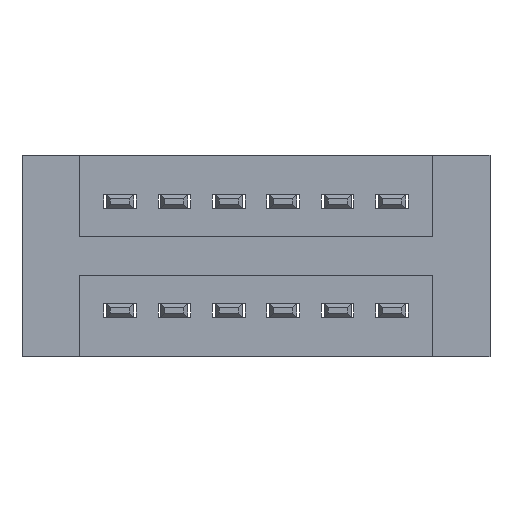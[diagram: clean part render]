
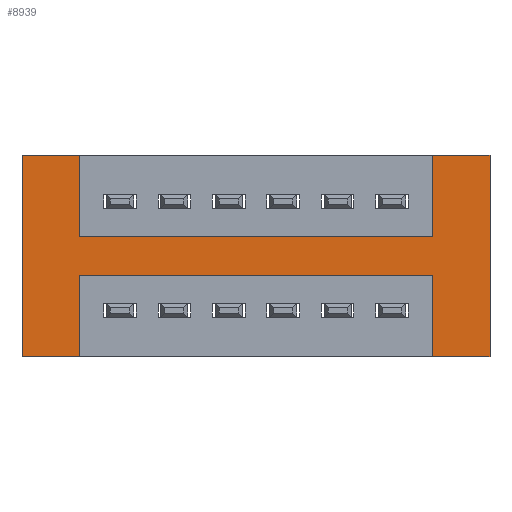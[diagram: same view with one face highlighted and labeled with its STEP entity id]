
A CAD part, front view. The second image highlights one B-rep face of the part: STEP entity #8939.
In plain terms, the highlighted planar face has unit normal (0, -1, 0).
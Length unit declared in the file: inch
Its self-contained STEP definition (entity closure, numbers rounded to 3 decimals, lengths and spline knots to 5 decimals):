
#86 = DIRECTION ( 'NONE',  ( 0., 0., -1. ) ) ;
#334 = DIRECTION ( 'NONE',  ( -1., 0., 0. ) ) ;
#479 = CARTESIAN_POINT ( 'NONE',  ( 0.3925, 0., -0.22 ) ) ;
#517 = VECTOR ( 'NONE', #3859, 39.37008 ) ;
#543 = ORIENTED_EDGE ( 'NONE', *, *, #7268, .F. ) ;
#548 = VECTOR ( 'NONE', #3588, 39.37008 ) ;
#1015 = VERTEX_POINT ( 'NONE', #8087 ) ;
#1110 = VERTEX_POINT ( 'NONE', #8718 ) ;
#1115 = VERTEX_POINT ( 'NONE', #8397 ) ;
#1174 = EDGE_CURVE ( 'NONE', #3664, #2440, #4881, .T. ) ;
#1403 = DIRECTION ( 'NONE',  ( 1., 0., 0. ) ) ;
#1459 = CARTESIAN_POINT ( 'NONE',  ( 1.0425, 0., -0.15 ) ) ;
#1495 = DIRECTION ( 'NONE',  ( 0., 0., 1. ) ) ;
#1603 = LINE ( 'NONE', #7203, #3324 ) ;
#1618 = LINE ( 'NONE', #4018, #8876 ) ;
#1695 = EDGE_CURVE ( 'NONE', #1115, #5210, #6433, .T. ) ;
#1724 = VERTEX_POINT ( 'NONE', #1761 ) ;
#1759 = DIRECTION ( 'NONE',  ( 0., 0., 1. ) ) ;
#1761 = CARTESIAN_POINT ( 'NONE',  ( 0.3925, 0., -0.37 ) ) ;
#1949 = EDGE_CURVE ( 'NONE', #2984, #5186, #8240, .T. ) ;
#2087 = EDGE_CURVE ( 'NONE', #5186, #4849, #5267, .T. ) ;
#2100 = VECTOR ( 'NONE', #8294, 39.37008 ) ;
#2111 = LINE ( 'NONE', #3970, #517 ) ;
#2144 = PLANE ( 'NONE',  #7568 ) ;
#2212 = VECTOR ( 'NONE', #3057, 39.37008 ) ;
#2410 = CARTESIAN_POINT ( 'NONE',  ( 0.3925, 0., -0.37 ) ) ;
#2432 = LINE ( 'NONE', #2410, #2212 ) ;
#2440 = VERTEX_POINT ( 'NONE', #5871 ) ;
#2491 = ORIENTED_EDGE ( 'NONE', *, *, #7507, .F. ) ;
#2665 = VERTEX_POINT ( 'NONE', #4403 ) ;
#2682 = CARTESIAN_POINT ( 'NONE',  ( 1.0425, 0., 0. ) ) ;
#2783 = CARTESIAN_POINT ( 'NONE',  ( 1.1475, 0., 0. ) ) ;
#2894 = DIRECTION ( 'NONE',  ( -1., 0., 0. ) ) ;
#2984 = VERTEX_POINT ( 'NONE', #5282 ) ;
#3057 = DIRECTION ( 'NONE',  ( 0., 0., -1. ) ) ;
#3156 = VECTOR ( 'NONE', #9092, 39.37008 ) ;
#3324 = VECTOR ( 'NONE', #2894, 39.37008 ) ;
#3435 = LINE ( 'NONE', #5165, #7123 ) ;
#3456 = ORIENTED_EDGE ( 'NONE', *, *, #1695, .T. ) ;
#3588 = DIRECTION ( 'NONE',  ( 0., 0., -1. ) ) ;
#3597 = CARTESIAN_POINT ( 'NONE',  ( 0., 0., -0.37 ) ) ;
#3601 = ORIENTED_EDGE ( 'NONE', *, *, #1174, .F. ) ;
#3664 = VERTEX_POINT ( 'NONE', #6521 ) ;
#3859 = DIRECTION ( 'NONE',  ( -1., 0., 0. ) ) ;
#3878 = CARTESIAN_POINT ( 'NONE',  ( 0.2875, 0., 0. ) ) ;
#3962 = VERTEX_POINT ( 'NONE', #2783 ) ;
#3970 = CARTESIAN_POINT ( 'NONE',  ( 0., 0., -0.37 ) ) ;
#4006 = LINE ( 'NONE', #7448, #2100 ) ;
#4018 = CARTESIAN_POINT ( 'NONE',  ( 0., 0., 0. ) ) ;
#4068 = EDGE_CURVE ( 'NONE', #2665, #3962, #3435, .T. ) ;
#4316 = EDGE_CURVE ( 'NONE', #1015, #1110, #1603, .T. ) ;
#4321 = DIRECTION ( 'NONE',  ( 0., 0., -1. ) ) ;
#4389 = VECTOR ( 'NONE', #86, 39.37008 ) ;
#4403 = CARTESIAN_POINT ( 'NONE',  ( 1.0425, 0., 0. ) ) ;
#4555 = CARTESIAN_POINT ( 'NONE',  ( 0.3925, 0., 0. ) ) ;
#4571 = ORIENTED_EDGE ( 'NONE', *, *, #8590, .T. ) ;
#4849 = VERTEX_POINT ( 'NONE', #1459 ) ;
#4881 = LINE ( 'NONE', #479, #6021 ) ;
#4915 = ORIENTED_EDGE ( 'NONE', *, *, #4316, .F. ) ;
#5067 = ORIENTED_EDGE ( 'NONE', *, *, #7570, .F. ) ;
#5124 = LINE ( 'NONE', #6022, #7116 ) ;
#5126 = EDGE_LOOP ( 'NONE', ( #4571, #5311, #7017, #7155, #8003, #5067, #3456, #6161, #543, #3601, #2491, #4915 ) ) ;
#5165 = CARTESIAN_POINT ( 'NONE',  ( 0., 0., 0. ) ) ;
#5186 = VERTEX_POINT ( 'NONE', #8872 ) ;
#5210 = VERTEX_POINT ( 'NONE', #8797 ) ;
#5267 = LINE ( 'NONE', #5527, #3156 ) ;
#5282 = CARTESIAN_POINT ( 'NONE',  ( 0.3925, 0., 0. ) ) ;
#5311 = ORIENTED_EDGE ( 'NONE', *, *, #4068, .F. ) ;
#5527 = CARTESIAN_POINT ( 'NONE',  ( 0.3925, 0., -0.15 ) ) ;
#5529 = EDGE_CURVE ( 'NONE', #4849, #2665, #7380, .T. ) ;
#5579 = VECTOR ( 'NONE', #1495, 39.37008 ) ;
#5736 = FACE_OUTER_BOUND ( 'NONE', #5126, .T. ) ;
#5871 = CARTESIAN_POINT ( 'NONE',  ( 0.3925, 0., -0.22 ) ) ;
#6021 = VECTOR ( 'NONE', #334, 39.37008 ) ;
#6022 = CARTESIAN_POINT ( 'NONE',  ( 1.1475, 0., 0. ) ) ;
#6161 = ORIENTED_EDGE ( 'NONE', *, *, #7076, .F. ) ;
#6433 = LINE ( 'NONE', #3878, #4389 ) ;
#6521 = CARTESIAN_POINT ( 'NONE',  ( 1.0425, 0., -0.22 ) ) ;
#7017 = ORIENTED_EDGE ( 'NONE', *, *, #5529, .F. ) ;
#7076 = EDGE_CURVE ( 'NONE', #1724, #5210, #2111, .T. ) ;
#7116 = VECTOR ( 'NONE', #1759, 39.37008 ) ;
#7123 = VECTOR ( 'NONE', #1403, 39.37008 ) ;
#7155 = ORIENTED_EDGE ( 'NONE', *, *, #2087, .F. ) ;
#7203 = CARTESIAN_POINT ( 'NONE',  ( 0., 0., -0.37 ) ) ;
#7268 = EDGE_CURVE ( 'NONE', #2440, #1724, #2432, .T. ) ;
#7380 = LINE ( 'NONE', #2682, #5579 ) ;
#7448 = CARTESIAN_POINT ( 'NONE',  ( 1.0425, 0., -0.37 ) ) ;
#7507 = EDGE_CURVE ( 'NONE', #1110, #3664, #4006, .T. ) ;
#7568 = AXIS2_PLACEMENT_3D ( 'NONE', #3597, #8309, #4321 ) ;
#7570 = EDGE_CURVE ( 'NONE', #1115, #2984, #1618, .T. ) ;
#8003 = ORIENTED_EDGE ( 'NONE', *, *, #1949, .F. ) ;
#8087 = CARTESIAN_POINT ( 'NONE',  ( 1.1475, 0., -0.37 ) ) ;
#8240 = LINE ( 'NONE', #4555, #548 ) ;
#8294 = DIRECTION ( 'NONE',  ( 0., 0., 1. ) ) ;
#8309 = DIRECTION ( 'NONE',  ( 0., -1., 0. ) ) ;
#8397 = CARTESIAN_POINT ( 'NONE',  ( 0.2875, 0., 0. ) ) ;
#8590 = EDGE_CURVE ( 'NONE', #1015, #3962, #5124, .T. ) ;
#8679 = DIRECTION ( 'NONE',  ( 1., 0., 0. ) ) ;
#8718 = CARTESIAN_POINT ( 'NONE',  ( 1.0425, 0., -0.37 ) ) ;
#8797 = CARTESIAN_POINT ( 'NONE',  ( 0.2875, 0., -0.37 ) ) ;
#8872 = CARTESIAN_POINT ( 'NONE',  ( 0.3925, 0., -0.15 ) ) ;
#8876 = VECTOR ( 'NONE', #8679, 39.37008 ) ;
#8939 = ADVANCED_FACE ( 'NONE', ( #5736 ), #2144, .T. ) ;
#9092 = DIRECTION ( 'NONE',  ( 1., 0., 0. ) ) ;
